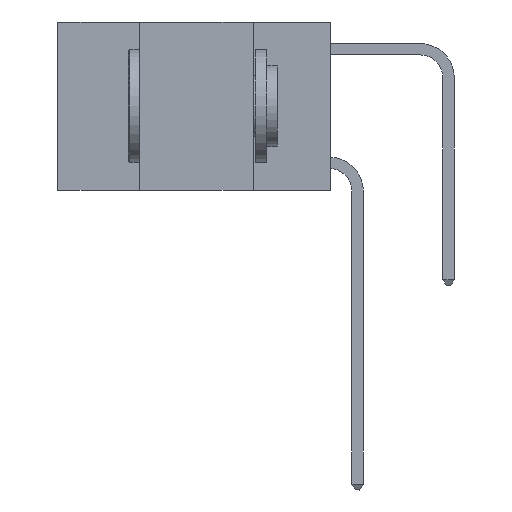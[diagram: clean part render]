
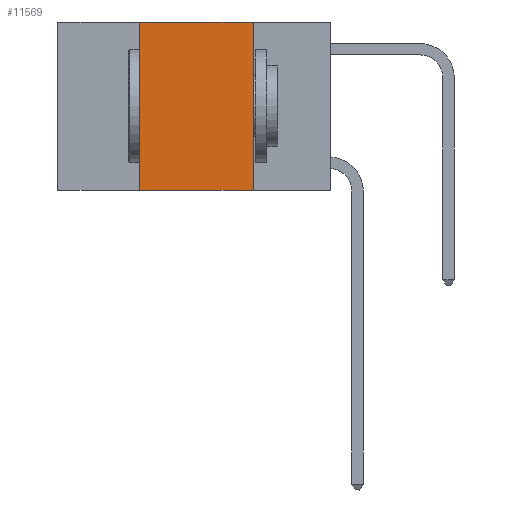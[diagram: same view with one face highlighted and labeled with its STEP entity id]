
A CAD part, left-side view. The second image highlights one B-rep face of the part: STEP entity #11569.
In plain terms, the highlighted planar face has unit normal (-1, 0, 0).
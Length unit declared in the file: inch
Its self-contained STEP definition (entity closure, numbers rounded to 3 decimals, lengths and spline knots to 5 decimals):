
#540 = CARTESIAN_POINT ( 'NONE',  ( 0., 0.42, 0. ) ) ;
#784 = LINE ( 'NONE', #19781, #11967 ) ;
#956 = PLANE ( 'NONE',  #19438 ) ;
#1315 = ORIENTED_EDGE ( 'NONE', *, *, #15259, .F. ) ;
#1384 = VERTEX_POINT ( 'NONE', #540 ) ;
#2298 = VECTOR ( 'NONE', #3806, 39.37008 ) ;
#2537 = LINE ( 'NONE', #17687, #2298 ) ;
#2753 = DIRECTION ( 'NONE',  ( 0., -1., 0. ) ) ;
#3540 = ORIENTED_EDGE ( 'NONE', *, *, #18197, .T. ) ;
#3688 = VERTEX_POINT ( 'NONE', #8982 ) ;
#3806 = DIRECTION ( 'NONE',  ( 0., 0., 1. ) ) ;
#4847 = FACE_OUTER_BOUND ( 'NONE', #12362, .T. ) ;
#7069 = CARTESIAN_POINT ( 'NONE',  ( 0., 0.6, 0. ) ) ;
#8834 = EDGE_CURVE ( 'NONE', #1384, #3688, #784, .T. ) ;
#8982 = CARTESIAN_POINT ( 'NONE',  ( 0., 0.17, 0. ) ) ;
#9264 = CARTESIAN_POINT ( 'NONE',  ( 0., 0.6, -0.37 ) ) ;
#9312 = LINE ( 'NONE', #12587, #9558 ) ;
#9558 = VECTOR ( 'NONE', #15718, 39.37008 ) ;
#11569 = ADVANCED_FACE ( 'NONE', ( #4847 ), #956, .F. ) ;
#11967 = VECTOR ( 'NONE', #11977, 39.37008 ) ;
#11977 = DIRECTION ( 'NONE',  ( 0., -1., 0. ) ) ;
#12023 = VERTEX_POINT ( 'NONE', #16034 ) ;
#12183 = VERTEX_POINT ( 'NONE', #14393 ) ;
#12362 = EDGE_LOOP ( 'NONE', ( #1315, #14017, #19384, #3540 ) ) ;
#12363 = VECTOR ( 'NONE', #2753, 39.37008 ) ;
#12587 = CARTESIAN_POINT ( 'NONE',  ( 0., 0.17, 0. ) ) ;
#14017 = ORIENTED_EDGE ( 'NONE', *, *, #8834, .F. ) ;
#14115 = EDGE_CURVE ( 'NONE', #12023, #1384, #2537, .T. ) ;
#14393 = CARTESIAN_POINT ( 'NONE',  ( 0., 0.17, -0.37 ) ) ;
#15259 = EDGE_CURVE ( 'NONE', #3688, #12183, #9312, .T. ) ;
#15718 = DIRECTION ( 'NONE',  ( 0., 0., -1. ) ) ;
#16034 = CARTESIAN_POINT ( 'NONE',  ( 0., 0.42, -0.37 ) ) ;
#17005 = LINE ( 'NONE', #9264, #12363 ) ;
#17687 = CARTESIAN_POINT ( 'NONE',  ( 0., 0.42, 0. ) ) ;
#17954 = DIRECTION ( 'NONE',  ( 0., 0., -1. ) ) ;
#18197 = EDGE_CURVE ( 'NONE', #12023, #12183, #17005, .T. ) ;
#19384 = ORIENTED_EDGE ( 'NONE', *, *, #14115, .F. ) ;
#19438 = AXIS2_PLACEMENT_3D ( 'NONE', #7069, #19538, #17954 ) ;
#19538 = DIRECTION ( 'NONE',  ( 1., 0., 0. ) ) ;
#19781 = CARTESIAN_POINT ( 'NONE',  ( 0., 0.6, 0. ) ) ;
